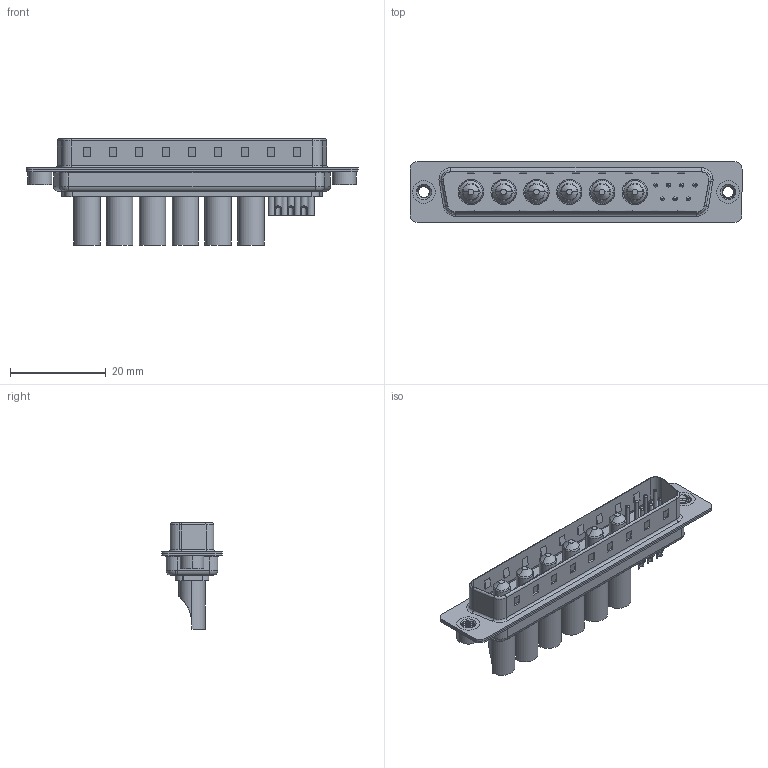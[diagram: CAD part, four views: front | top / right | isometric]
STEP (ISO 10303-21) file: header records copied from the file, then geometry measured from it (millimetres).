
FILE_DESCRIPTION (( 'STEP AP203' ), '1' );
FILE_NAME ('627-13W6622-4NA.STEP', '2019-05-28T21:23:24', ( '' ), ( '' ), 'SwSTEP 2.0', 'SolidWorks 2016', '' );
FILE_SCHEMA (( 'CONFIG_CONTROL_DESIGN' ));
Length unit declared in the file: millimetre
Products named in the file (9): 627Combo Threaded Rivet_2; 627Combo Contact Row 1_22; 627Combo Contact Row 2_22; 627-13W6622-4NA; 627Combo Housing_13W6; 627Combo Shell Rear_37 Contacts; 627Combo Shell Front_37 Contacts; 627Combo Threaded Rivet_A; Power Pin_40A SC
Assembly tree (18 placements, depth 2):
  627-13W6622-4NA
    627Combo Housing_13W6
    627Combo Shell Rear_37 Contacts
    627Combo Shell Front_37 Contacts
    627Combo Threaded Rivet_A
    Power Pin_40A SC  x6
    627Combo Threaded Rivet_2
    627Combo Contact Row 1_22  x4
    627Combo Contact Row 2_22  x3
Bounding box: 69.3 x 12.6 x 22.3 mm (x, y, z)
Volume: 4431.1 mm3; surface area: 9957.8 mm2
Topology: 24 solids, 24 shells, 928 faces, 2218 edges, 1363 vertices
Faces by surface type: cylinder 374, plane 338, torus 132, cone 66, bspline 18
Entity records: 22159 total; most frequent: CARTESIAN_POINT 6530, DIRECTION 3126, ORIENTED_EDGE 2920, EDGE_CURVE 1460, AXIS2_PLACEMENT_3D 1167, VERTEX_POINT 923, VECTOR 792, LINE 792
